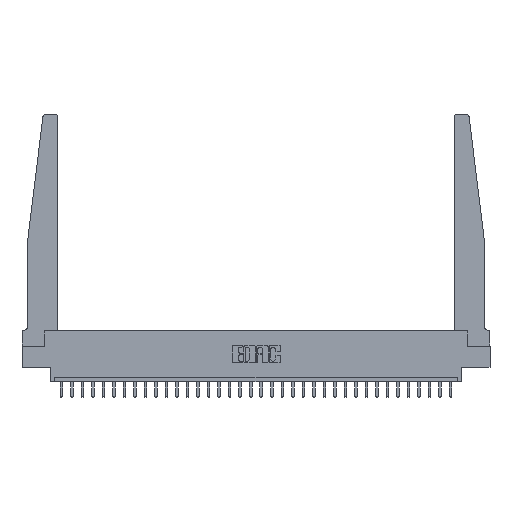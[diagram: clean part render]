
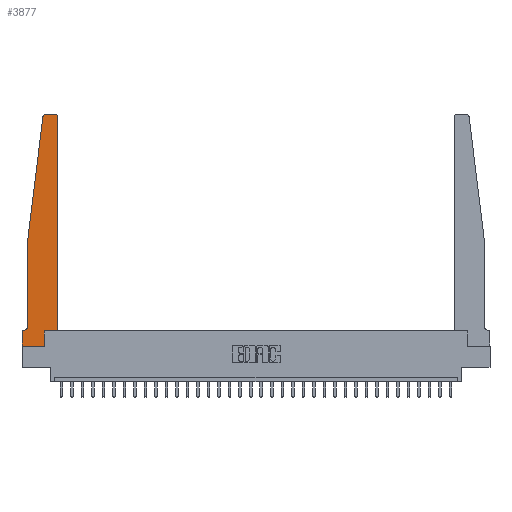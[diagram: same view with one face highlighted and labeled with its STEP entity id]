
A CAD part, top view. The second image highlights one B-rep face of the part: STEP entity #3877.
In plain terms, the highlighted planar face has unit normal (0, 0, 1).
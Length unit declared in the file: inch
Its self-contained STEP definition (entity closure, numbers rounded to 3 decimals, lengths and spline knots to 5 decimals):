
#193 = VECTOR ( 'NONE', #20370, 39.37008 ) ;
#234 = VERTEX_POINT ( 'NONE', #18223 ) ;
#395 = DIRECTION ( 'NONE',  ( 1., 0., 0. ) ) ;
#666 = ORIENTED_EDGE ( 'NONE', *, *, #5143, .T. ) ;
#931 = CARTESIAN_POINT ( 'NONE',  ( 0.065, 1.25, 0.37 ) ) ;
#942 = VERTEX_POINT ( 'NONE', #17226 ) ;
#1702 = DIRECTION ( 'NONE',  ( 0., 0., 1. ) ) ;
#2560 = CARTESIAN_POINT ( 'NONE',  ( 0., 0., 0.37 ) ) ;
#2609 = CARTESIAN_POINT ( 'NONE',  ( 0.27653, 2.75, 0.37 ) ) ;
#2649 = AXIS2_PLACEMENT_3D ( 'NONE', #18402, #4910, #22907 ) ;
#2660 = DIRECTION ( 'NONE',  ( 0., 0., 1. ) ) ;
#2710 = LINE ( 'NONE', #11097, #24860 ) ;
#2784 = VERTEX_POINT ( 'NONE', #9880 ) ;
#3877 = ADVANCED_FACE ( 'NONE', ( #27801 ), #24337, .T. ) ;
#3938 = CARTESIAN_POINT ( 'NONE',  ( 0.395, 2.72, 0.37 ) ) ;
#3951 = LINE ( 'NONE', #4573, #16949 ) ;
#4257 = CARTESIAN_POINT ( 'NONE',  ( 0.25, 2.75, 0.37 ) ) ;
#4516 = LINE ( 'NONE', #931, #13635 ) ;
#4553 = DIRECTION ( 'NONE',  ( -1., 0., 0. ) ) ;
#4573 = CARTESIAN_POINT ( 'NONE',  ( 0.065, 1.25, 0.37 ) ) ;
#4910 = DIRECTION ( 'NONE',  ( 0., 0., -1. ) ) ;
#5143 = EDGE_CURVE ( 'NONE', #942, #28313, #4516, .T. ) ;
#5748 = CIRCLE ( 'NONE', #18193, 0.03 ) ;
#6214 = EDGE_CURVE ( 'NONE', #234, #2784, #6527, .T. ) ;
#6364 = ORIENTED_EDGE ( 'NONE', *, *, #27395, .T. ) ;
#6448 = DIRECTION ( 'NONE',  ( 0., 0., 1. ) ) ;
#6527 = LINE ( 'NONE', #9421, #193 ) ;
#6565 = DIRECTION ( 'NONE',  ( 0., 1., 0. ) ) ;
#7081 = LINE ( 'NONE', #2560, #13421 ) ;
#7454 = EDGE_CURVE ( 'NONE', #9819, #13938, #5748, .T. ) ;
#7562 = ORIENTED_EDGE ( 'NONE', *, *, #25269, .T. ) ;
#8441 = EDGE_CURVE ( 'NONE', #14680, #22778, #23723, .T. ) ;
#9067 = CARTESIAN_POINT ( 'NONE',  ( 0.065, 0.1875, 0.37 ) ) ;
#9421 = CARTESIAN_POINT ( 'NONE',  ( 0., 0., 0.37 ) ) ;
#9819 = VERTEX_POINT ( 'NONE', #2609 ) ;
#9880 = CARTESIAN_POINT ( 'NONE',  ( 0.2605, 0., 0.37 ) ) ;
#9961 = VECTOR ( 'NONE', #13759, 39.37008 ) ;
#10066 = VECTOR ( 'NONE', #4553, 39.37008 ) ;
#10103 = CARTESIAN_POINT ( 'NONE',  ( 0.425, 2.72, 0.37 ) ) ;
#10442 = DIRECTION ( 'NONE',  ( 0., 1., 0. ) ) ;
#10548 = CARTESIAN_POINT ( 'NONE',  ( 0.425, 0.18, 0.37 ) ) ;
#10639 = ORIENTED_EDGE ( 'NONE', *, *, #19856, .T. ) ;
#10779 = CARTESIAN_POINT ( 'NONE',  ( 0.425, 0.18, 0.37 ) ) ;
#10988 = DIRECTION ( 'NONE',  ( 1., 0., 0. ) ) ;
#11097 = CARTESIAN_POINT ( 'NONE',  ( 0.2605, 0.18, 0.37 ) ) ;
#11146 = CARTESIAN_POINT ( 'NONE',  ( 0.395, 2.75, 0.37 ) ) ;
#11569 = CARTESIAN_POINT ( 'NONE',  ( 0.015, 0.1875, 0.37 ) ) ;
#12315 = DIRECTION ( 'NONE',  ( 0., -1., 0. ) ) ;
#12786 = EDGE_CURVE ( 'NONE', #2784, #14680, #2710, .T. ) ;
#12858 = VERTEX_POINT ( 'NONE', #11569 ) ;
#13421 = VECTOR ( 'NONE', #22729, 39.37008 ) ;
#13624 = VECTOR ( 'NONE', #10442, 39.37008 ) ;
#13635 = VECTOR ( 'NONE', #12315, 39.37008 ) ;
#13759 = DIRECTION ( 'NONE',  ( 1., 0., 0. ) ) ;
#13938 = VERTEX_POINT ( 'NONE', #24603 ) ;
#14220 = LINE ( 'NONE', #4257, #24087 ) ;
#14680 = VERTEX_POINT ( 'NONE', #25209 ) ;
#15173 = CARTESIAN_POINT ( 'NONE',  ( 0., 0.1875, 0.37 ) ) ;
#16022 = CARTESIAN_POINT ( 'NONE',  ( 0., 0.1875, 0.37 ) ) ;
#16335 = ORIENTED_EDGE ( 'NONE', *, *, #27264, .T. ) ;
#16474 = ORIENTED_EDGE ( 'NONE', *, *, #22868, .T. ) ;
#16942 = VERTEX_POINT ( 'NONE', #16022 ) ;
#16949 = VECTOR ( 'NONE', #27179, 39.37008 ) ;
#17226 = CARTESIAN_POINT ( 'NONE',  ( 0.065, 1.25, 0.37 ) ) ;
#17440 = DIRECTION ( 'NONE',  ( 1., 0., 0. ) ) ;
#18193 = AXIS2_PLACEMENT_3D ( 'NONE', #24801, #2660, #395 ) ;
#18223 = CARTESIAN_POINT ( 'NONE',  ( 0., 0., 0.37 ) ) ;
#18253 = ORIENTED_EDGE ( 'NONE', *, *, #8441, .T. ) ;
#18402 = CARTESIAN_POINT ( 'NONE',  ( 0.015, 0.2375, 0.37 ) ) ;
#18518 = CARTESIAN_POINT ( 'NONE',  ( 0.425, 0.18, 0.37 ) ) ;
#18834 = ORIENTED_EDGE ( 'NONE', *, *, #7454, .T. ) ;
#19225 = AXIS2_PLACEMENT_3D ( 'NONE', #3938, #6448, #10988 ) ;
#19816 = ORIENTED_EDGE ( 'NONE', *, *, #12786, .T. ) ;
#19856 = EDGE_CURVE ( 'NONE', #12858, #16942, #23470, .T. ) ;
#20370 = DIRECTION ( 'NONE',  ( 1., 0., 0. ) ) ;
#20680 = CIRCLE ( 'NONE', #2649, 0.05 ) ;
#21218 = CARTESIAN_POINT ( 'NONE',  ( 0.065, 0.2375, 0.37 ) ) ;
#22134 = EDGE_CURVE ( 'NONE', #27648, #24795, #26183, .T. ) ;
#22243 = EDGE_LOOP ( 'NONE', ( #16335, #18834, #16474, #666, #23280, #10639, #6364, #25898, #19816, #18253, #7562, #22997 ) ) ;
#22254 = DIRECTION ( 'NONE',  ( -1., 0., 0. ) ) ;
#22729 = DIRECTION ( 'NONE',  ( 0., -1., 0. ) ) ;
#22778 = VERTEX_POINT ( 'NONE', #10779 ) ;
#22868 = EDGE_CURVE ( 'NONE', #13938, #942, #3951, .T. ) ;
#22907 = DIRECTION ( 'NONE',  ( -1., 0., 0. ) ) ;
#22997 = ORIENTED_EDGE ( 'NONE', *, *, #22134, .T. ) ;
#23280 = ORIENTED_EDGE ( 'NONE', *, *, #25479, .T. ) ;
#23470 = LINE ( 'NONE', #9067, #10066 ) ;
#23568 = AXIS2_PLACEMENT_3D ( 'NONE', #15173, #1702, #17440 ) ;
#23723 = LINE ( 'NONE', #18518, #9961 ) ;
#24087 = VECTOR ( 'NONE', #22254, 39.37008 ) ;
#24337 = PLANE ( 'NONE',  #23568 ) ;
#24603 = CARTESIAN_POINT ( 'NONE',  ( 0.24675, 2.72367, 0.37 ) ) ;
#24795 = VERTEX_POINT ( 'NONE', #11146 ) ;
#24801 = CARTESIAN_POINT ( 'NONE',  ( 0.27653, 2.72, 0.37 ) ) ;
#24860 = VECTOR ( 'NONE', #6565, 39.37008 ) ;
#25209 = CARTESIAN_POINT ( 'NONE',  ( 0.2605, 0.18, 0.37 ) ) ;
#25269 = EDGE_CURVE ( 'NONE', #22778, #27648, #28070, .T. ) ;
#25479 = EDGE_CURVE ( 'NONE', #28313, #12858, #20680, .T. ) ;
#25898 = ORIENTED_EDGE ( 'NONE', *, *, #6214, .T. ) ;
#26183 = CIRCLE ( 'NONE', #19225, 0.03 ) ;
#27179 = DIRECTION ( 'NONE',  ( -0.122, -0.992, 0. ) ) ;
#27264 = EDGE_CURVE ( 'NONE', #24795, #9819, #14220, .T. ) ;
#27395 = EDGE_CURVE ( 'NONE', #16942, #234, #7081, .T. ) ;
#27648 = VERTEX_POINT ( 'NONE', #10103 ) ;
#27801 = FACE_OUTER_BOUND ( 'NONE', #22243, .T. ) ;
#28070 = LINE ( 'NONE', #10548, #13624 ) ;
#28313 = VERTEX_POINT ( 'NONE', #21218 ) ;
